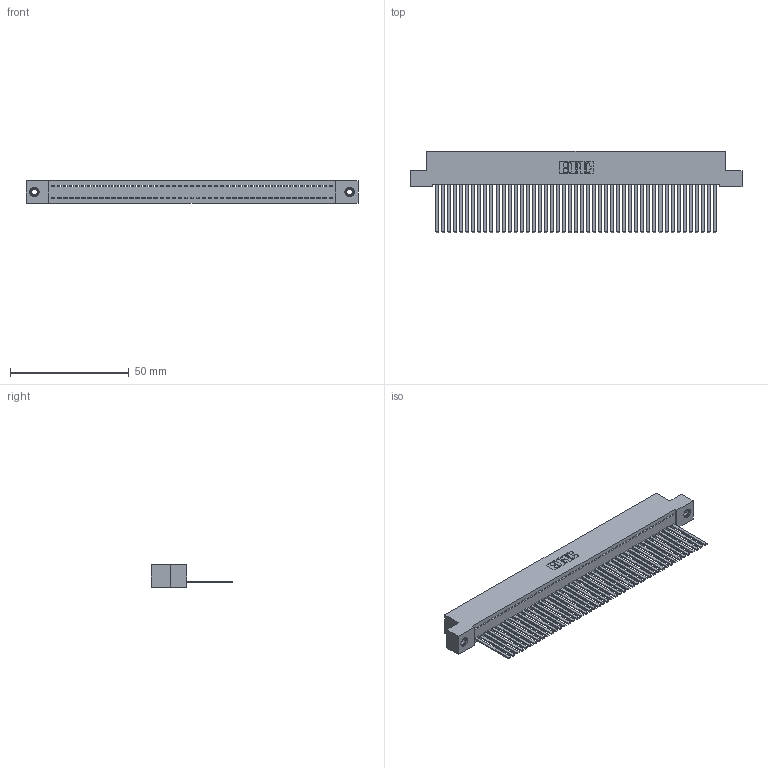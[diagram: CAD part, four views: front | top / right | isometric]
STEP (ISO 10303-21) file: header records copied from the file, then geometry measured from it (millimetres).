
FILE_DESCRIPTION (( 'STEP AP203' ), '1' );
FILE_NAME ('392-047-544-107.STEP', '2019-10-08T00:32:35', ( '' ), ( '' ), 'SwSTEP 2.0', 'SolidWorks 2016', '' );
FILE_SCHEMA (( 'CONFIG_CONTROL_DESIGN' ));
Length unit declared in the file: inch
Products named in the file (4): 342 Part_TI; 345-292-001_345-293-144; 345-250-001_345-250-005-103; 392-047-544-107
Assembly tree (50 placements, depth 2):
  392-047-544-107
    342 Part_TI
    345-292-001_345-293-144  x47
    345-250-001_345-250-005-103  x2
Bounding box: 139.7 x 34.3 x 9.4 mm (x, y, z)
Volume: 12798.9 mm3; surface area: 20469.4 mm2
Topology: 50 solids, 50 shells, 2614 faces, 7861 edges, 5170 vertices
Faces by surface type: plane 1884, cylinder 714, cone 12, torus 4
Entity records: 28956 total; most frequent: CARTESIAN_POINT 4974, ORIENTED_EDGE 4950, DIRECTION 4215, EDGE_CURVE 2475, VECTOR 2331, LINE 2331, VERTEX_POINT 1644, AXIS2_PLACEMENT_3D 942
